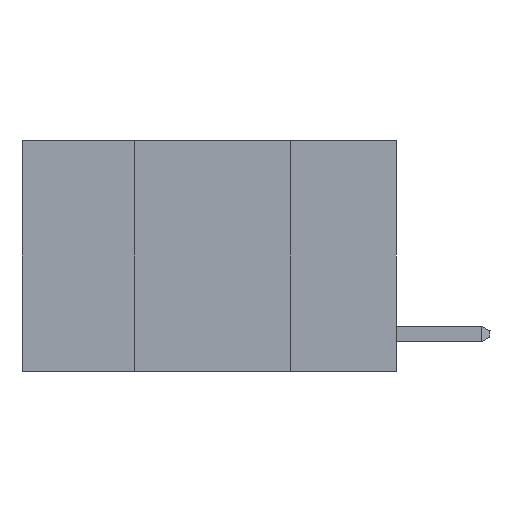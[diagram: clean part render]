
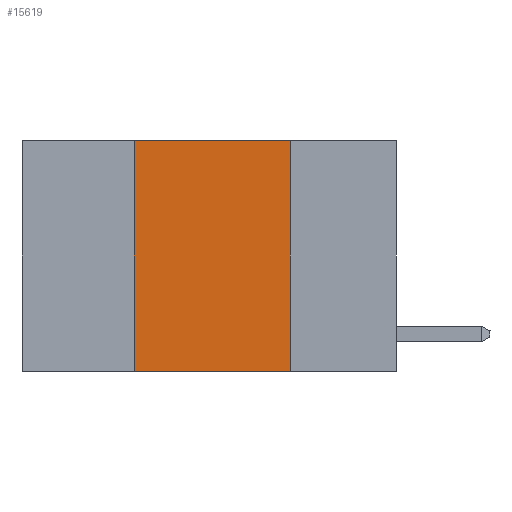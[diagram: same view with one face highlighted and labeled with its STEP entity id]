
A CAD part, left-side view. The second image highlights one B-rep face of the part: STEP entity #15619.
In plain terms, the highlighted planar face has unit normal (-1, 0, 0).
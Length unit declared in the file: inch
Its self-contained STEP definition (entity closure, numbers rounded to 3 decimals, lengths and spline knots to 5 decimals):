
#122 = VERTEX_POINT ( 'NONE', #10935 ) ;
#1145 = EDGE_CURVE ( 'NONE', #3213, #14036, #8302, .T. ) ;
#2133 = VERTEX_POINT ( 'NONE', #17491 ) ;
#2719 = CARTESIAN_POINT ( 'NONE',  ( 0., 0.42, -0.37 ) ) ;
#3213 = VERTEX_POINT ( 'NONE', #2719 ) ;
#3235 = DIRECTION ( 'NONE',  ( 0., 0., -1. ) ) ;
#5737 = FACE_OUTER_BOUND ( 'NONE', #15366, .T. ) ;
#5957 = CARTESIAN_POINT ( 'NONE',  ( 0., 0.17, 0. ) ) ;
#6224 = PLANE ( 'NONE',  #12575 ) ;
#6328 = LINE ( 'NONE', #5957, #14369 ) ;
#6418 = CARTESIAN_POINT ( 'NONE',  ( 0., 0.6, -0.37 ) ) ;
#8302 = LINE ( 'NONE', #17764, #8976 ) ;
#8976 = VECTOR ( 'NONE', #9296, 39.37008 ) ;
#8991 = DIRECTION ( 'NONE',  ( 1., 0., 0. ) ) ;
#9103 = DIRECTION ( 'NONE',  ( 0., 0., -1. ) ) ;
#9296 = DIRECTION ( 'NONE',  ( 0., 0., 1. ) ) ;
#9457 = LINE ( 'NONE', #6418, #12364 ) ;
#10159 = ORIENTED_EDGE ( 'NONE', *, *, #11945, .F. ) ;
#10204 = CARTESIAN_POINT ( 'NONE',  ( 0., 0.42, 0. ) ) ;
#10935 = CARTESIAN_POINT ( 'NONE',  ( 0., 0.17, 0. ) ) ;
#11945 = EDGE_CURVE ( 'NONE', #122, #2133, #6328, .T. ) ;
#12364 = VECTOR ( 'NONE', #17060, 39.37008 ) ;
#12394 = ORIENTED_EDGE ( 'NONE', *, *, #1145, .F. ) ;
#12575 = AXIS2_PLACEMENT_3D ( 'NONE', #17758, #8991, #9103 ) ;
#12629 = ORIENTED_EDGE ( 'NONE', *, *, #17645, .F. ) ;
#13917 = LINE ( 'NONE', #18288, #16363 ) ;
#14036 = VERTEX_POINT ( 'NONE', #10204 ) ;
#14183 = DIRECTION ( 'NONE',  ( 0., -1., 0. ) ) ;
#14238 = ORIENTED_EDGE ( 'NONE', *, *, #17075, .T. ) ;
#14369 = VECTOR ( 'NONE', #3235, 39.37008 ) ;
#15366 = EDGE_LOOP ( 'NONE', ( #10159, #12629, #12394, #14238 ) ) ;
#15619 = ADVANCED_FACE ( 'NONE', ( #5737 ), #6224, .F. ) ;
#16363 = VECTOR ( 'NONE', #14183, 39.37008 ) ;
#17060 = DIRECTION ( 'NONE',  ( 0., -1., 0. ) ) ;
#17075 = EDGE_CURVE ( 'NONE', #3213, #2133, #9457, .T. ) ;
#17491 = CARTESIAN_POINT ( 'NONE',  ( 0., 0.17, -0.37 ) ) ;
#17645 = EDGE_CURVE ( 'NONE', #14036, #122, #13917, .T. ) ;
#17758 = CARTESIAN_POINT ( 'NONE',  ( 0., 0.6, 0. ) ) ;
#17764 = CARTESIAN_POINT ( 'NONE',  ( 0., 0.42, 0. ) ) ;
#18288 = CARTESIAN_POINT ( 'NONE',  ( 0., 0.6, 0. ) ) ;
